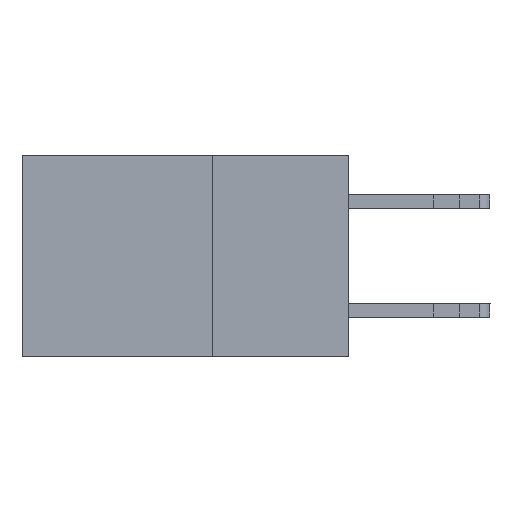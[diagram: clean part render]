
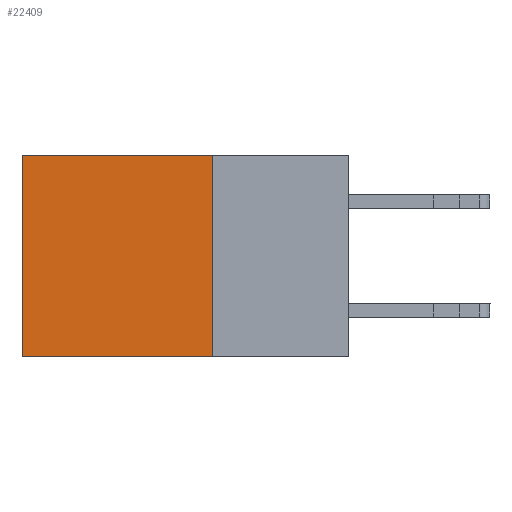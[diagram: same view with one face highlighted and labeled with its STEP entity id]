
A CAD part, left-side view. The second image highlights one B-rep face of the part: STEP entity #22409.
In plain terms, the highlighted planar face has unit normal (-1, 0, 0).
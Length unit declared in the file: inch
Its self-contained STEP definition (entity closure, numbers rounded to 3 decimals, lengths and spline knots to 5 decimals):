
#941 = ORIENTED_EDGE ( 'NONE', *, *, #11864, .T. ) ;
#1443 = CARTESIAN_POINT ( 'NONE',  ( 0.2615, 0.25, -0.37 ) ) ;
#2057 = DIRECTION ( 'NONE',  ( 0., 1., 0. ) ) ;
#2145 = CARTESIAN_POINT ( 'NONE',  ( 0.2615, 0.6, -0.37 ) ) ;
#2795 = EDGE_CURVE ( 'NONE', #12013, #11601, #12713, .T. ) ;
#3940 = DIRECTION ( 'NONE',  ( 0., 0., -1. ) ) ;
#6908 = VECTOR ( 'NONE', #20402, 39.37008 ) ;
#7142 = CARTESIAN_POINT ( 'NONE',  ( 0.2615, 0.25, -0.37 ) ) ;
#7454 = LINE ( 'NONE', #8927, #20146 ) ;
#7728 = DIRECTION ( 'NONE',  ( 0., 0., -1. ) ) ;
#8193 = CARTESIAN_POINT ( 'NONE',  ( 0.2615, 0.6, 0. ) ) ;
#8927 = CARTESIAN_POINT ( 'NONE',  ( 0.2615, 0.25, 0. ) ) ;
#9427 = DIRECTION ( 'NONE',  ( 1., 0., 0. ) ) ;
#9647 = LINE ( 'NONE', #2145, #13713 ) ;
#10131 = EDGE_LOOP ( 'NONE', ( #12472, #17788, #17302, #941 ) ) ;
#10246 = CARTESIAN_POINT ( 'NONE',  ( 0.2615, 0.6, -0.37 ) ) ;
#11125 = VERTEX_POINT ( 'NONE', #10246 ) ;
#11479 = LINE ( 'NONE', #11725, #6908 ) ;
#11516 = VERTEX_POINT ( 'NONE', #8193 ) ;
#11601 = VERTEX_POINT ( 'NONE', #1443 ) ;
#11725 = CARTESIAN_POINT ( 'NONE',  ( 0.2615, 0.25, -0.37 ) ) ;
#11864 = EDGE_CURVE ( 'NONE', #12013, #11516, #7454, .T. ) ;
#12013 = VERTEX_POINT ( 'NONE', #12810 ) ;
#12297 = EDGE_CURVE ( 'NONE', #11601, #11125, #11479, .T. ) ;
#12472 = ORIENTED_EDGE ( 'NONE', *, *, #17336, .T. ) ;
#12713 = LINE ( 'NONE', #7142, #13258 ) ;
#12810 = CARTESIAN_POINT ( 'NONE',  ( 0.2615, 0.25, 0. ) ) ;
#13258 = VECTOR ( 'NONE', #7728, 39.37008 ) ;
#13713 = VECTOR ( 'NONE', #3940, 39.37008 ) ;
#16308 = CARTESIAN_POINT ( 'NONE',  ( 0.2615, 0.25, -0.37 ) ) ;
#17302 = ORIENTED_EDGE ( 'NONE', *, *, #2795, .F. ) ;
#17336 = EDGE_CURVE ( 'NONE', #11516, #11125, #9647, .T. ) ;
#17788 = ORIENTED_EDGE ( 'NONE', *, *, #12297, .F. ) ;
#18887 = FACE_OUTER_BOUND ( 'NONE', #10131, .T. ) ;
#19377 = AXIS2_PLACEMENT_3D ( 'NONE', #16308, #9427, #21502 ) ;
#19792 = PLANE ( 'NONE',  #19377 ) ;
#20146 = VECTOR ( 'NONE', #2057, 39.37008 ) ;
#20402 = DIRECTION ( 'NONE',  ( 0., 1., 0. ) ) ;
#21502 = DIRECTION ( 'NONE',  ( 0., 0., -1. ) ) ;
#22409 = ADVANCED_FACE ( 'NONE', ( #18887 ), #19792, .F. ) ;
